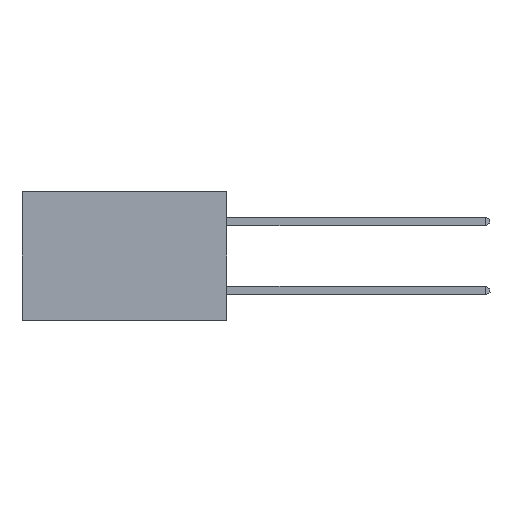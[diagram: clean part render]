
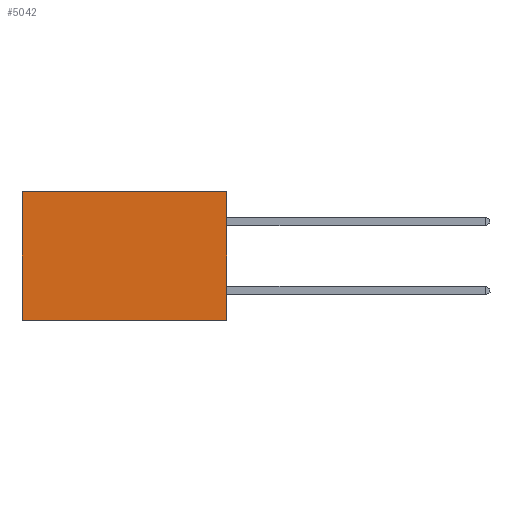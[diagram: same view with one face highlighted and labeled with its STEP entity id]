
A CAD part, left-side view. The second image highlights one B-rep face of the part: STEP entity #5042.
In plain terms, the highlighted planar face has unit normal (-1, 0, 0).
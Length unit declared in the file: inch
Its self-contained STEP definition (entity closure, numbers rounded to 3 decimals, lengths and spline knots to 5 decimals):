
#436 = EDGE_CURVE ( 'NONE', #2392, #8225, #5320, .T. ) ;
#666 = EDGE_CURVE ( 'NONE', #8225, #6448, #2216, .T. ) ;
#864 = CARTESIAN_POINT ( 'NONE',  ( 0.277, 0.59, -0.37 ) ) ;
#1104 = DIRECTION ( 'NONE',  ( 0., 0., -1. ) ) ;
#1138 = DIRECTION ( 'NONE',  ( 0., 1., 0. ) ) ;
#2125 = EDGE_CURVE ( 'NONE', #2633, #6448, #9193, .T. ) ;
#2141 = EDGE_CURVE ( 'NONE', #2392, #2633, #5854, .T. ) ;
#2216 = LINE ( 'NONE', #864, #9138 ) ;
#2392 = VERTEX_POINT ( 'NONE', #8280 ) ;
#2490 = CARTESIAN_POINT ( 'NONE',  ( 0.277, 0., 0. ) ) ;
#2633 = VERTEX_POINT ( 'NONE', #8014 ) ;
#2816 = VECTOR ( 'NONE', #8818, 39.37008 ) ;
#2961 = PLANE ( 'NONE',  #5350 ) ;
#3715 = DIRECTION ( 'NONE',  ( 0., 0., -1. ) ) ;
#3872 = DIRECTION ( 'NONE',  ( 0., 0., -1. ) ) ;
#5042 = ADVANCED_FACE ( 'NONE', ( #8163 ), #2961, .F. ) ;
#5320 = LINE ( 'NONE', #2490, #2816 ) ;
#5350 = AXIS2_PLACEMENT_3D ( 'NONE', #6597, #7878, #3715 ) ;
#5854 = LINE ( 'NONE', #9349, #7358 ) ;
#6448 = VERTEX_POINT ( 'NONE', #7122 ) ;
#6597 = CARTESIAN_POINT ( 'NONE',  ( 0.277, 0., -0.37 ) ) ;
#6827 = ORIENTED_EDGE ( 'NONE', *, *, #2141, .F. ) ;
#7078 = ORIENTED_EDGE ( 'NONE', *, *, #666, .T. ) ;
#7122 = CARTESIAN_POINT ( 'NONE',  ( 0.277, 0.59, -0.37 ) ) ;
#7250 = CARTESIAN_POINT ( 'NONE',  ( 0.277, 0., -0.37 ) ) ;
#7358 = VECTOR ( 'NONE', #1104, 39.37008 ) ;
#7572 = VECTOR ( 'NONE', #1138, 39.37008 ) ;
#7878 = DIRECTION ( 'NONE',  ( 1., 0., 0. ) ) ;
#8014 = CARTESIAN_POINT ( 'NONE',  ( 0.277, 0., -0.37 ) ) ;
#8163 = FACE_OUTER_BOUND ( 'NONE', #9046, .T. ) ;
#8225 = VERTEX_POINT ( 'NONE', #8618 ) ;
#8280 = CARTESIAN_POINT ( 'NONE',  ( 0.277, 0., 0. ) ) ;
#8417 = ORIENTED_EDGE ( 'NONE', *, *, #2125, .F. ) ;
#8618 = CARTESIAN_POINT ( 'NONE',  ( 0.277, 0.59, 0. ) ) ;
#8818 = DIRECTION ( 'NONE',  ( 0., 1., 0. ) ) ;
#9046 = EDGE_LOOP ( 'NONE', ( #7078, #8417, #6827, #9216 ) ) ;
#9138 = VECTOR ( 'NONE', #3872, 39.37008 ) ;
#9193 = LINE ( 'NONE', #7250, #7572 ) ;
#9216 = ORIENTED_EDGE ( 'NONE', *, *, #436, .T. ) ;
#9349 = CARTESIAN_POINT ( 'NONE',  ( 0.277, 0., -0.37 ) ) ;
